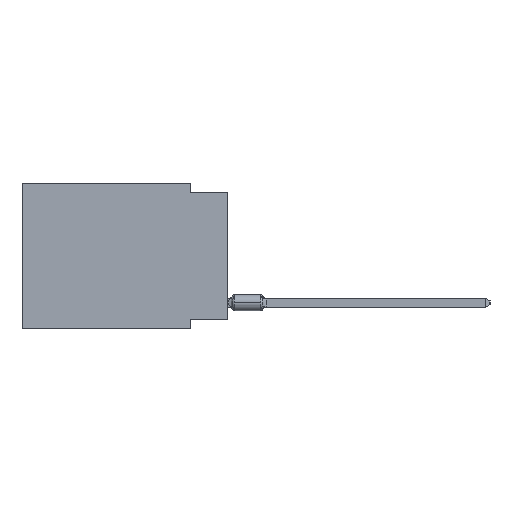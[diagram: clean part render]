
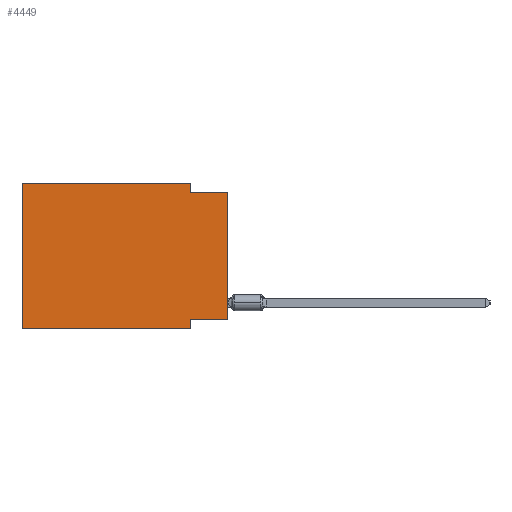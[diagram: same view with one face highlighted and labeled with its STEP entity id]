
A CAD part, left-side view. The second image highlights one B-rep face of the part: STEP entity #4449.
In plain terms, the highlighted planar face has unit normal (-1, 0, 0).
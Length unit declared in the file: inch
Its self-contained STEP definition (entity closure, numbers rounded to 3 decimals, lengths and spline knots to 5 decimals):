
#165 = VECTOR ( 'NONE', #1900, 39.37008 ) ;
#399 = CARTESIAN_POINT ( 'NONE',  ( 0., 0.1, -0.39 ) ) ;
#508 = LINE ( 'NONE', #8050, #13616 ) ;
#616 = LINE ( 'NONE', #3187, #165 ) ;
#832 = ORIENTED_EDGE ( 'NONE', *, *, #10833, .F. ) ;
#955 = VERTEX_POINT ( 'NONE', #15826 ) ;
#1100 = VECTOR ( 'NONE', #9824, 39.37008 ) ;
#1518 = CARTESIAN_POINT ( 'NONE',  ( 0., 0.1, -0.39 ) ) ;
#1561 = LINE ( 'NONE', #14919, #12437 ) ;
#1657 = EDGE_CURVE ( 'NONE', #16409, #955, #616, .T. ) ;
#1900 = DIRECTION ( 'NONE',  ( 0., 0., 1. ) ) ;
#2027 = VERTEX_POINT ( 'NONE', #7196 ) ;
#2480 = LINE ( 'NONE', #12836, #9315 ) ;
#3187 = CARTESIAN_POINT ( 'NONE',  ( 0., 0., 0. ) ) ;
#3253 = FACE_OUTER_BOUND ( 'NONE', #7812, .T. ) ;
#4449 = ADVANCED_FACE ( 'NONE', ( #3253 ), #11388, .F. ) ;
#4473 = DIRECTION ( 'NONE',  ( 0., 1., 0. ) ) ;
#5595 = EDGE_CURVE ( 'NONE', #16409, #15125, #1561, .T. ) ;
#5768 = CARTESIAN_POINT ( 'NONE',  ( 0., 0.55, -0.39 ) ) ;
#6326 = DIRECTION ( 'NONE',  ( 0., 0., 1. ) ) ;
#6555 = ORIENTED_EDGE ( 'NONE', *, *, #12800, .F. ) ;
#6785 = CARTESIAN_POINT ( 'NONE',  ( 0., 0.55, -0.39 ) ) ;
#6901 = ORIENTED_EDGE ( 'NONE', *, *, #16045, .F. ) ;
#7196 = CARTESIAN_POINT ( 'NONE',  ( 0., 0.1, 0. ) ) ;
#7285 = CARTESIAN_POINT ( 'NONE',  ( 0., 0., -0.025 ) ) ;
#7288 = EDGE_CURVE ( 'NONE', #7647, #955, #15067, .T. ) ;
#7519 = CARTESIAN_POINT ( 'NONE',  ( 0., 0.1, 0. ) ) ;
#7527 = CARTESIAN_POINT ( 'NONE',  ( 0., 0., -0.365 ) ) ;
#7647 = VERTEX_POINT ( 'NONE', #13589 ) ;
#7699 = VECTOR ( 'NONE', #12494, 39.37008 ) ;
#7812 = EDGE_LOOP ( 'NONE', ( #13443, #11735, #8689, #6555, #6901, #14607, #832, #11644 ) ) ;
#8050 = CARTESIAN_POINT ( 'NONE',  ( 0., 0.55, 0. ) ) ;
#8458 = VERTEX_POINT ( 'NONE', #6785 ) ;
#8524 = DIRECTION ( 'NONE',  ( 0., 0., -1. ) ) ;
#8578 = DIRECTION ( 'NONE',  ( 1., 0., 0. ) ) ;
#8689 = ORIENTED_EDGE ( 'NONE', *, *, #13591, .F. ) ;
#9243 = VERTEX_POINT ( 'NONE', #399 ) ;
#9315 = VECTOR ( 'NONE', #6326, 39.37008 ) ;
#9823 = VECTOR ( 'NONE', #14021, 39.37008 ) ;
#9824 = DIRECTION ( 'NONE',  ( 0., -1., 0. ) ) ;
#10414 = VERTEX_POINT ( 'NONE', #15915 ) ;
#10803 = VECTOR ( 'NONE', #8524, 39.37008 ) ;
#10833 = EDGE_CURVE ( 'NONE', #15125, #9243, #13242, .T. ) ;
#10876 = DIRECTION ( 'NONE',  ( 0., -1., 0. ) ) ;
#11388 = PLANE ( 'NONE',  #15884 ) ;
#11644 = ORIENTED_EDGE ( 'NONE', *, *, #5595, .F. ) ;
#11735 = ORIENTED_EDGE ( 'NONE', *, *, #7288, .F. ) ;
#12024 = LINE ( 'NONE', #5768, #1100 ) ;
#12437 = VECTOR ( 'NONE', #4473, 39.37008 ) ;
#12494 = DIRECTION ( 'NONE',  ( 0., -1., 0. ) ) ;
#12800 = EDGE_CURVE ( 'NONE', #10414, #2027, #508, .T. ) ;
#12836 = CARTESIAN_POINT ( 'NONE',  ( 0., 0.55, 0. ) ) ;
#13242 = LINE ( 'NONE', #1518, #10803 ) ;
#13443 = ORIENTED_EDGE ( 'NONE', *, *, #1657, .T. ) ;
#13589 = CARTESIAN_POINT ( 'NONE',  ( 0., 0.1, -0.025 ) ) ;
#13591 = EDGE_CURVE ( 'NONE', #2027, #7647, #15470, .T. ) ;
#13616 = VECTOR ( 'NONE', #10876, 39.37008 ) ;
#13833 = CARTESIAN_POINT ( 'NONE',  ( 0., 0.1, -0.365 ) ) ;
#14021 = DIRECTION ( 'NONE',  ( 0., 0., -1. ) ) ;
#14607 = ORIENTED_EDGE ( 'NONE', *, *, #14932, .T. ) ;
#14919 = CARTESIAN_POINT ( 'NONE',  ( 0., 0., -0.365 ) ) ;
#14932 = EDGE_CURVE ( 'NONE', #8458, #9243, #12024, .T. ) ;
#15067 = LINE ( 'NONE', #7285, #7699 ) ;
#15125 = VERTEX_POINT ( 'NONE', #13833 ) ;
#15152 = CARTESIAN_POINT ( 'NONE',  ( 0., 0.55, 0. ) ) ;
#15470 = LINE ( 'NONE', #7519, #9823 ) ;
#15826 = CARTESIAN_POINT ( 'NONE',  ( 0., 0., -0.025 ) ) ;
#15884 = AXIS2_PLACEMENT_3D ( 'NONE', #15152, #8578, #16267 ) ;
#15915 = CARTESIAN_POINT ( 'NONE',  ( 0., 0.55, 0. ) ) ;
#16045 = EDGE_CURVE ( 'NONE', #8458, #10414, #2480, .T. ) ;
#16267 = DIRECTION ( 'NONE',  ( 0., 0., -1. ) ) ;
#16409 = VERTEX_POINT ( 'NONE', #7527 ) ;
